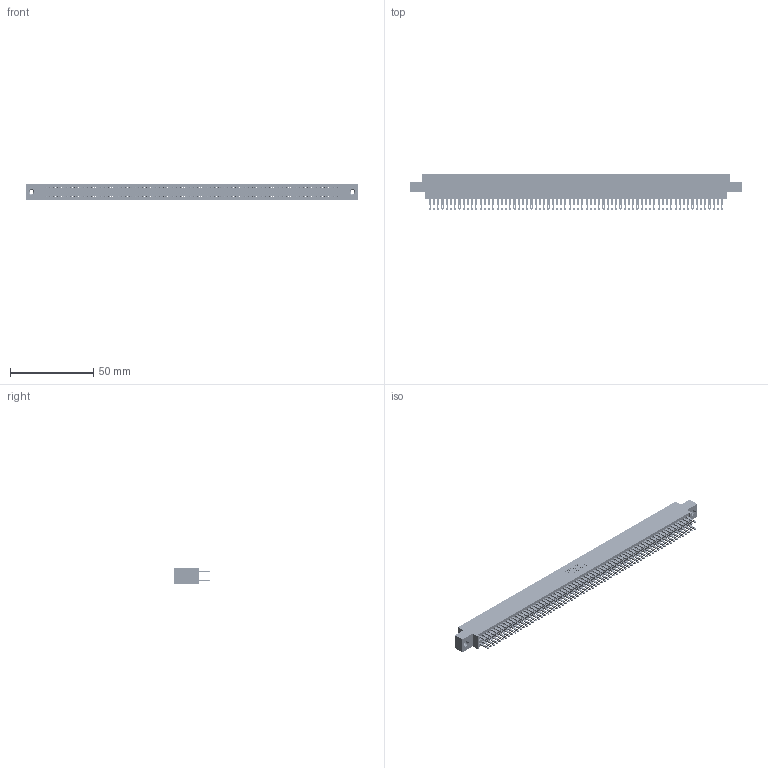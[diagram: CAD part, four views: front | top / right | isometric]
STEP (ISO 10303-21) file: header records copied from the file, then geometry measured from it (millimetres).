
FILE_DESCRIPTION (( 'STEP AP203' ), '1' );
FILE_NAME ('895-140-500-808.STEP', '2020-10-13T19:40:55', ( '' ), ( '' ), 'SwSTEP 2.0', 'SolidWorks 2020', '' );
FILE_SCHEMA (( 'CONFIG_CONTROL_DESIGN' ));
Length unit declared in the file: inch
Products named in the file (4): 345-250-001_345-250-003-102; 345-292-001_345-293-100; 895-140-500-808; 845 Part_0.170 Offset - 0.156 Dia-TI
Assembly tree (143 placements, depth 2):
  895-140-500-808
    845 Part_0.170 Offset - 0.156 Dia-TI
    345-292-001_345-293-100  x140
    345-250-001_345-250-003-102  x2
Bounding box: 199.01 x 21.51 x 9.4 mm (x, y, z)
Volume: 19899.8 mm3; surface area: 31542.3 mm2
Topology: 143 solids, 143 shells, 6630 faces, 20229 edges, 13478 vertices
Faces by surface type: plane 3896, cylinder 2718, cone 12, torus 4
Entity records: 52402 total; most frequent: CARTESIAN_POINT 8739, ORIENTED_EDGE 8666, DIRECTION 7699, EDGE_CURVE 4333, LINE 3897, VECTOR 3897, VERTEX_POINT 2884, AXIS2_PLACEMENT_3D 1901
